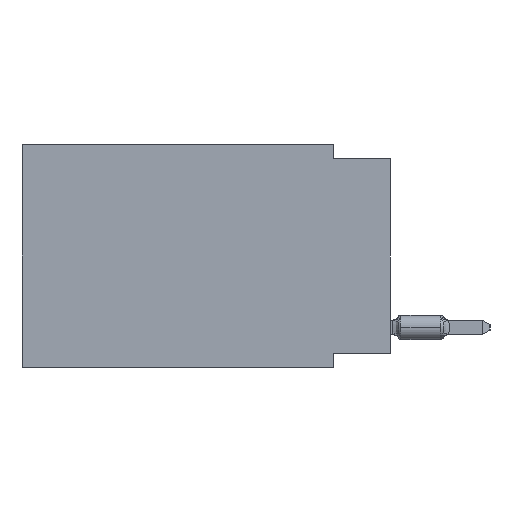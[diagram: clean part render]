
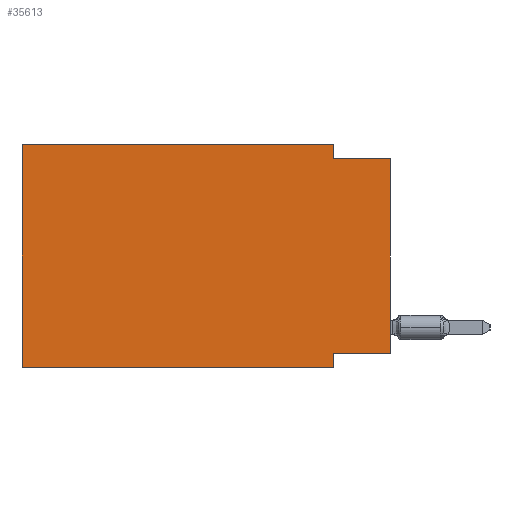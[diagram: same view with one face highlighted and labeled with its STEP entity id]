
A CAD part, left-side view. The second image highlights one B-rep face of the part: STEP entity #35613.
In plain terms, the highlighted planar face has unit normal (-1, 0, 0).
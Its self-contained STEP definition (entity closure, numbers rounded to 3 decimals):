
#547 = ORIENTED_EDGE ( 'NONE', *, *, #36082, .F. ) ;
#566 = LINE ( 'NONE', #8717, #82287 ) ;
#816 = EDGE_CURVE ( 'NONE', #83227, #16231, #28153, .T. ) ;
#2330 = ORIENTED_EDGE ( 'NONE', *, *, #15262, .F. ) ;
#4334 = DIRECTION ( 'NONE',  ( 0., 0., -1. ) ) ;
#4923 = ORIENTED_EDGE ( 'NONE', *, *, #27395, .T. ) ;
#5871 = DIRECTION ( 'NONE',  ( 1., 0., 0. ) ) ;
#6059 = LINE ( 'NONE', #19453, #25998 ) ;
#6315 = EDGE_CURVE ( 'NONE', #70489, #16231, #44880, .T. ) ;
#8717 = CARTESIAN_POINT ( 'NONE',  ( 0., 0., -0.635 ) ) ;
#9021 = VECTOR ( 'NONE', #41542, 1000. ) ;
#11124 = LINE ( 'NONE', #76751, #77804 ) ;
#12628 = ORIENTED_EDGE ( 'NONE', *, *, #6315, .F. ) ;
#13924 = EDGE_CURVE ( 'NONE', #82404, #21256, #15011, .T. ) ;
#15011 = LINE ( 'NONE', #28382, #37600 ) ;
#15262 = EDGE_CURVE ( 'NONE', #42248, #70489, #11124, .T. ) ;
#16125 = CARTESIAN_POINT ( 'NONE',  ( 0., 2.54, 0. ) ) ;
#16231 = VERTEX_POINT ( 'NONE', #57597 ) ;
#16301 = DIRECTION ( 'NONE',  ( 0., 1., 0. ) ) ;
#16351 = LINE ( 'NONE', #49574, #45522 ) ;
#18307 = ORIENTED_EDGE ( 'NONE', *, *, #30354, .F. ) ;
#19453 = CARTESIAN_POINT ( 'NONE',  ( 0., 16.383, 0. ) ) ;
#19631 = ORIENTED_EDGE ( 'NONE', *, *, #56825, .F. ) ;
#21256 = VERTEX_POINT ( 'NONE', #81909 ) ;
#22017 = VECTOR ( 'NONE', #4334, 1000. ) ;
#22916 = AXIS2_PLACEMENT_3D ( 'NONE', #38646, #5871, #32152 ) ;
#25583 = CARTESIAN_POINT ( 'NONE',  ( 0., 0., -9.271 ) ) ;
#25998 = VECTOR ( 'NONE', #39265, 1000. ) ;
#27395 = EDGE_CURVE ( 'NONE', #42248, #83790, #16351, .T. ) ;
#27553 = DIRECTION ( 'NONE',  ( 0., 0., -1. ) ) ;
#28153 = LINE ( 'NONE', #54918, #9021 ) ;
#28382 = CARTESIAN_POINT ( 'NONE',  ( 0., 2.54, 0. ) ) ;
#30354 = EDGE_CURVE ( 'NONE', #83227, #85160, #32198, .T. ) ;
#31481 = CARTESIAN_POINT ( 'NONE',  ( 0., 2.54, -9.906 ) ) ;
#32152 = DIRECTION ( 'NONE',  ( 0., 0., -1. ) ) ;
#32198 = LINE ( 'NONE', #51648, #34865 ) ;
#34512 = ORIENTED_EDGE ( 'NONE', *, *, #816, .T. ) ;
#34865 = VECTOR ( 'NONE', #65067, 1000. ) ;
#34999 = DIRECTION ( 'NONE',  ( 0., -1., 0. ) ) ;
#35613 = ADVANCED_FACE ( 'NONE', ( #77977 ), #45121, .F. ) ;
#36082 = EDGE_CURVE ( 'NONE', #21256, #83790, #566, .T. ) ;
#37600 = VECTOR ( 'NONE', #27553, 1000. ) ;
#38646 = CARTESIAN_POINT ( 'NONE',  ( 0., 16.383, 0. ) ) ;
#38921 = CARTESIAN_POINT ( 'NONE',  ( 0., 2.54, -9.271 ) ) ;
#39265 = DIRECTION ( 'NONE',  ( 0., -1., 0. ) ) ;
#41542 = DIRECTION ( 'NONE',  ( 0., -1., 0. ) ) ;
#42248 = VERTEX_POINT ( 'NONE', #25583 ) ;
#43179 = ORIENTED_EDGE ( 'NONE', *, *, #13924, .F. ) ;
#43398 = CARTESIAN_POINT ( 'NONE',  ( 0., 16.383, -9.906 ) ) ;
#44180 = CARTESIAN_POINT ( 'NONE',  ( 0., 0., -0.635 ) ) ;
#44880 = LINE ( 'NONE', #31481, #22017 ) ;
#45121 = PLANE ( 'NONE',  #22916 ) ;
#45522 = VECTOR ( 'NONE', #75085, 1000. ) ;
#49574 = CARTESIAN_POINT ( 'NONE',  ( 0., 0., 0. ) ) ;
#51648 = CARTESIAN_POINT ( 'NONE',  ( 0., 16.383, 0. ) ) ;
#53645 = CARTESIAN_POINT ( 'NONE',  ( 0., 16.383, 0. ) ) ;
#54918 = CARTESIAN_POINT ( 'NONE',  ( 0., 16.383, -9.906 ) ) ;
#54965 = EDGE_LOOP ( 'NONE', ( #4923, #547, #43179, #19631, #18307, #34512, #12628, #2330 ) ) ;
#56825 = EDGE_CURVE ( 'NONE', #85160, #82404, #6059, .T. ) ;
#57597 = CARTESIAN_POINT ( 'NONE',  ( 0., 2.54, -9.906 ) ) ;
#65067 = DIRECTION ( 'NONE',  ( 0., 0., 1. ) ) ;
#70489 = VERTEX_POINT ( 'NONE', #38921 ) ;
#75085 = DIRECTION ( 'NONE',  ( 0., 0., 1. ) ) ;
#76751 = CARTESIAN_POINT ( 'NONE',  ( 0., 0., -9.271 ) ) ;
#77804 = VECTOR ( 'NONE', #16301, 1000. ) ;
#77977 = FACE_OUTER_BOUND ( 'NONE', #54965, .T. ) ;
#81909 = CARTESIAN_POINT ( 'NONE',  ( 0., 2.54, -0.635 ) ) ;
#82287 = VECTOR ( 'NONE', #34999, 1000. ) ;
#82404 = VERTEX_POINT ( 'NONE', #16125 ) ;
#83227 = VERTEX_POINT ( 'NONE', #43398 ) ;
#83790 = VERTEX_POINT ( 'NONE', #44180 ) ;
#85160 = VERTEX_POINT ( 'NONE', #53645 ) ;
